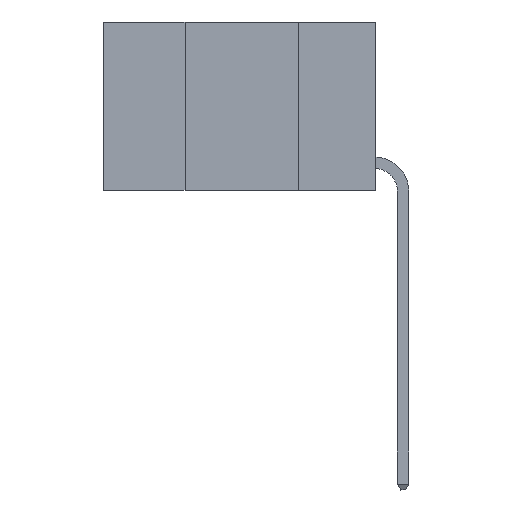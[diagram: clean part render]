
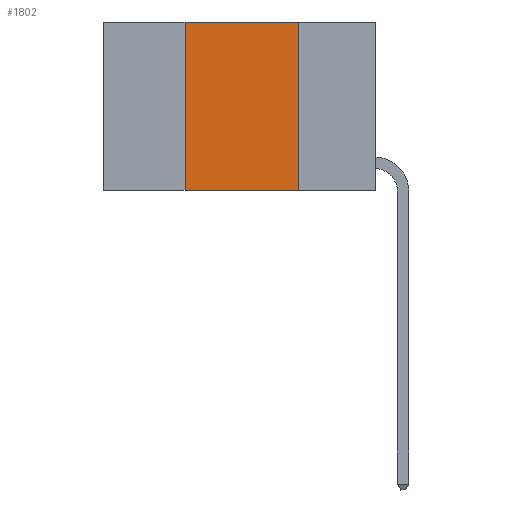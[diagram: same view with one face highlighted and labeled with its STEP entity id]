
A CAD part, left-side view. The second image highlights one B-rep face of the part: STEP entity #1802.
In plain terms, the highlighted planar face has unit normal (-1, 0, 0).
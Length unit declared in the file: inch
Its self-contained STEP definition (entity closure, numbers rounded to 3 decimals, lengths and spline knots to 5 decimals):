
#188 = CARTESIAN_POINT ( 'NONE',  ( 0., 0.17, 0. ) ) ;
#208 = VECTOR ( 'NONE', #5542, 39.37008 ) ;
#547 = CARTESIAN_POINT ( 'NONE',  ( 0., 0.42, 0. ) ) ;
#1169 = VERTEX_POINT ( 'NONE', #8055 ) ;
#1253 = EDGE_LOOP ( 'NONE', ( #6619, #7646, #6024, #10113 ) ) ;
#1802 = ADVANCED_FACE ( 'NONE', ( #9969 ), #3548, .F. ) ;
#2342 = CARTESIAN_POINT ( 'NONE',  ( 0., 0.42, 0. ) ) ;
#2667 = DIRECTION ( 'NONE',  ( 0., -1., 0. ) ) ;
#3343 = CARTESIAN_POINT ( 'NONE',  ( 0., 0.17, 0. ) ) ;
#3461 = LINE ( 'NONE', #3343, #4817 ) ;
#3548 = PLANE ( 'NONE',  #3854 ) ;
#3854 = AXIS2_PLACEMENT_3D ( 'NONE', #6459, #10161, #7248 ) ;
#3883 = VECTOR ( 'NONE', #8908, 39.37008 ) ;
#3972 = CARTESIAN_POINT ( 'NONE',  ( 0., 0.42, -0.37 ) ) ;
#3974 = EDGE_CURVE ( 'NONE', #10566, #9012, #9293, .T. ) ;
#4486 = EDGE_CURVE ( 'NONE', #9012, #1169, #3461, .T. ) ;
#4817 = VECTOR ( 'NONE', #11749, 39.37008 ) ;
#5542 = DIRECTION ( 'NONE',  ( 0., -1., 0. ) ) ;
#6024 = ORIENTED_EDGE ( 'NONE', *, *, #8723, .F. ) ;
#6052 = LINE ( 'NONE', #547, #3883 ) ;
#6215 = EDGE_CURVE ( 'NONE', #7076, #1169, #11107, .T. ) ;
#6459 = CARTESIAN_POINT ( 'NONE',  ( 0., 0.6, 0. ) ) ;
#6619 = ORIENTED_EDGE ( 'NONE', *, *, #4486, .F. ) ;
#7076 = VERTEX_POINT ( 'NONE', #3972 ) ;
#7248 = DIRECTION ( 'NONE',  ( 0., 0., -1. ) ) ;
#7338 = CARTESIAN_POINT ( 'NONE',  ( 0., 0.6, 0. ) ) ;
#7426 = CARTESIAN_POINT ( 'NONE',  ( 0., 0.6, -0.37 ) ) ;
#7646 = ORIENTED_EDGE ( 'NONE', *, *, #3974, .F. ) ;
#8055 = CARTESIAN_POINT ( 'NONE',  ( 0., 0.17, -0.37 ) ) ;
#8723 = EDGE_CURVE ( 'NONE', #7076, #10566, #6052, .T. ) ;
#8908 = DIRECTION ( 'NONE',  ( 0., 0., 1. ) ) ;
#9012 = VERTEX_POINT ( 'NONE', #188 ) ;
#9293 = LINE ( 'NONE', #7338, #10023 ) ;
#9969 = FACE_OUTER_BOUND ( 'NONE', #1253, .T. ) ;
#10023 = VECTOR ( 'NONE', #2667, 39.37008 ) ;
#10113 = ORIENTED_EDGE ( 'NONE', *, *, #6215, .T. ) ;
#10161 = DIRECTION ( 'NONE',  ( 1., 0., 0. ) ) ;
#10566 = VERTEX_POINT ( 'NONE', #2342 ) ;
#11107 = LINE ( 'NONE', #7426, #208 ) ;
#11749 = DIRECTION ( 'NONE',  ( 0., 0., -1. ) ) ;
